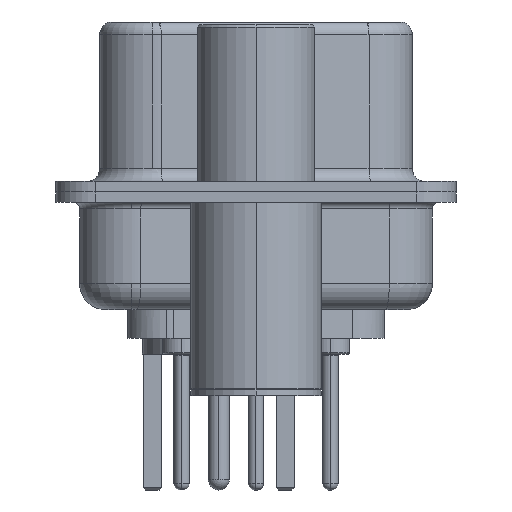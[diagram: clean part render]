
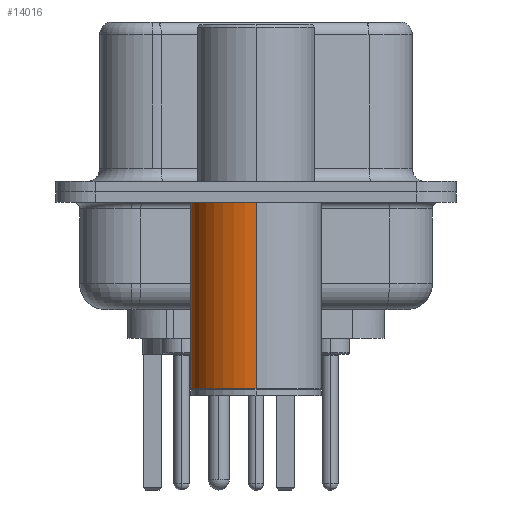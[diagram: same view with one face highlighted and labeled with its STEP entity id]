
A CAD part, left-side view. The second image highlights one B-rep face of the part: STEP entity #14016.
In plain terms, the highlighted cylindrical face has radius 2.5 mm (diameter 5 mm), a partial arc.
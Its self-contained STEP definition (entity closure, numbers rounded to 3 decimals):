
#1783 = CARTESIAN_POINT ( 'NONE',  ( -2.5, 0., 0.581 ) ) ;
#1964 = CARTESIAN_POINT ( 'NONE',  ( 2.5, 0., -0.4 ) ) ;
#2453 = VECTOR ( 'NONE', #21927, 1000. ) ;
#3520 = CARTESIAN_POINT ( 'NONE',  ( 0., 0., -7.525 ) ) ;
#3523 = AXIS2_PLACEMENT_3D ( 'NONE', #4956, #25514, #7866 ) ;
#4308 = FACE_OUTER_BOUND ( 'NONE', #17635, .T. ) ;
#4956 = CARTESIAN_POINT ( 'NONE',  ( 0., 0., -0.4 ) ) ;
#6411 = DIRECTION ( 'NONE',  ( 1., 0., 0. ) ) ;
#7866 = DIRECTION ( 'NONE',  ( 1., 0., 0. ) ) ;
#8356 = ORIENTED_EDGE ( 'NONE', *, *, #24179, .F. ) ;
#8652 = VERTEX_POINT ( 'NONE', #21148 ) ;
#9229 = CIRCLE ( 'NONE', #15649, 2.5 ) ;
#9254 = LINE ( 'NONE', #27797, #2453 ) ;
#9741 = CARTESIAN_POINT ( 'NONE',  ( 2.5, 0., -7.525 ) ) ;
#9788 = VERTEX_POINT ( 'NONE', #1964 ) ;
#13001 = DIRECTION ( 'NONE',  ( 1., 0., 0. ) ) ;
#14016 = ADVANCED_FACE ( 'NONE', ( #4308 ), #18080, .T. ) ;
#15649 = AXIS2_PLACEMENT_3D ( 'NONE', #3520, #24058, #6411 ) ;
#15719 = VECTOR ( 'NONE', #22356, 1000. ) ;
#17218 = ORIENTED_EDGE ( 'NONE', *, *, #36657, .T. ) ;
#17578 = VERTEX_POINT ( 'NONE', #9741 ) ;
#17635 = EDGE_LOOP ( 'NONE', ( #27074, #17218, #20554, #8356 ) ) ;
#18080 = CYLINDRICAL_SURFACE ( 'NONE', #18667, 2.5 ) ;
#18512 = VERTEX_POINT ( 'NONE', #32172 ) ;
#18667 = AXIS2_PLACEMENT_3D ( 'NONE', #33374, #30573, #13001 ) ;
#20554 = ORIENTED_EDGE ( 'NONE', *, *, #35069, .F. ) ;
#21148 = CARTESIAN_POINT ( 'NONE',  ( -2.5, 0., -0.4 ) ) ;
#21927 = DIRECTION ( 'NONE',  ( 0., 0., 1. ) ) ;
#22356 = DIRECTION ( 'NONE',  ( 0., 0., 1. ) ) ;
#24058 = DIRECTION ( 'NONE',  ( 0., 0., 1. ) ) ;
#24179 = EDGE_CURVE ( 'NONE', #17578, #9788, #9254, .T. ) ;
#25514 = DIRECTION ( 'NONE',  ( 0., 0., 1. ) ) ;
#27074 = ORIENTED_EDGE ( 'NONE', *, *, #35796, .T. ) ;
#27797 = CARTESIAN_POINT ( 'NONE',  ( 2.5, 0., 0.581 ) ) ;
#30367 = LINE ( 'NONE', #1783, #15719 ) ;
#30573 = DIRECTION ( 'NONE',  ( 0., 0., 1. ) ) ;
#32172 = CARTESIAN_POINT ( 'NONE',  ( -2.5, 0., -7.525 ) ) ;
#33374 = CARTESIAN_POINT ( 'NONE',  ( 0., 0., 0.581 ) ) ;
#35069 = EDGE_CURVE ( 'NONE', #9788, #8652, #36394, .T. ) ;
#35796 = EDGE_CURVE ( 'NONE', #17578, #18512, #9229, .T. ) ;
#36394 = CIRCLE ( 'NONE', #3523, 2.5 ) ;
#36657 = EDGE_CURVE ( 'NONE', #18512, #8652, #30367, .T. ) ;
